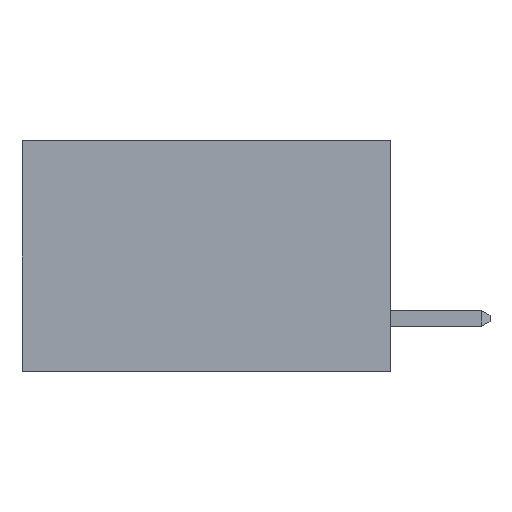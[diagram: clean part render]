
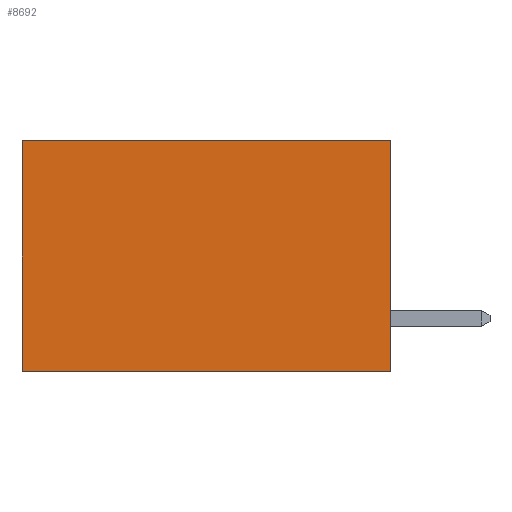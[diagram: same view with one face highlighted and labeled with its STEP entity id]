
A CAD part, left-side view. The second image highlights one B-rep face of the part: STEP entity #8692.
In plain terms, the highlighted planar face has unit normal (-1, 0, 0).
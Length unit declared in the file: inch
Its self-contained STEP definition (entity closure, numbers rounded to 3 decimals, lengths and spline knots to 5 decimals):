
#1019 = DIRECTION ( 'NONE',  ( 0., 1., 0. ) ) ;
#1155 = CARTESIAN_POINT ( 'NONE',  ( 0.277, 0.59, -0.37 ) ) ;
#1341 = DIRECTION ( 'NONE',  ( 0., 0., -1. ) ) ;
#1480 = CARTESIAN_POINT ( 'NONE',  ( 0.277, 0.59, 0. ) ) ;
#1924 = VERTEX_POINT ( 'NONE', #8272 ) ;
#2374 = LINE ( 'NONE', #3578, #6251 ) ;
#2405 = CARTESIAN_POINT ( 'NONE',  ( 0.277, 0., -0.37 ) ) ;
#2700 = DIRECTION ( 'NONE',  ( 0., 1., 0. ) ) ;
#3157 = VECTOR ( 'NONE', #2700, 39.37008 ) ;
#3196 = DIRECTION ( 'NONE',  ( 0., 0., -1. ) ) ;
#3273 = LINE ( 'NONE', #5460, #7127 ) ;
#3347 = EDGE_LOOP ( 'NONE', ( #4886, #5008, #5987, #7467 ) ) ;
#3578 = CARTESIAN_POINT ( 'NONE',  ( 0.277, 0.59, -0.37 ) ) ;
#4511 = PLANE ( 'NONE',  #7831 ) ;
#4545 = DIRECTION ( 'NONE',  ( 0., 0., -1. ) ) ;
#4702 = FACE_OUTER_BOUND ( 'NONE', #3347, .T. ) ;
#4886 = ORIENTED_EDGE ( 'NONE', *, *, #7751, .T. ) ;
#5008 = ORIENTED_EDGE ( 'NONE', *, *, #8138, .F. ) ;
#5043 = LINE ( 'NONE', #7020, #3157 ) ;
#5460 = CARTESIAN_POINT ( 'NONE',  ( 0.277, 0., -0.37 ) ) ;
#5473 = VERTEX_POINT ( 'NONE', #1155 ) ;
#5987 = ORIENTED_EDGE ( 'NONE', *, *, #8732, .F. ) ;
#6251 = VECTOR ( 'NONE', #1341, 39.37008 ) ;
#6695 = LINE ( 'NONE', #7525, #8296 ) ;
#7020 = CARTESIAN_POINT ( 'NONE',  ( 0.277, 0., 0. ) ) ;
#7127 = VECTOR ( 'NONE', #1019, 39.37008 ) ;
#7467 = ORIENTED_EDGE ( 'NONE', *, *, #8935, .T. ) ;
#7525 = CARTESIAN_POINT ( 'NONE',  ( 0.277, 0., -0.37 ) ) ;
#7751 = EDGE_CURVE ( 'NONE', #9218, #5473, #2374, .T. ) ;
#7831 = AXIS2_PLACEMENT_3D ( 'NONE', #2405, #8795, #4545 ) ;
#8038 = CARTESIAN_POINT ( 'NONE',  ( 0.277, 0., 0. ) ) ;
#8138 = EDGE_CURVE ( 'NONE', #1924, #5473, #3273, .T. ) ;
#8272 = CARTESIAN_POINT ( 'NONE',  ( 0.277, 0., -0.37 ) ) ;
#8296 = VECTOR ( 'NONE', #3196, 39.37008 ) ;
#8586 = VERTEX_POINT ( 'NONE', #8038 ) ;
#8692 = ADVANCED_FACE ( 'NONE', ( #4702 ), #4511, .F. ) ;
#8732 = EDGE_CURVE ( 'NONE', #8586, #1924, #6695, .T. ) ;
#8795 = DIRECTION ( 'NONE',  ( 1., 0., 0. ) ) ;
#8935 = EDGE_CURVE ( 'NONE', #8586, #9218, #5043, .T. ) ;
#9218 = VERTEX_POINT ( 'NONE', #1480 ) ;
